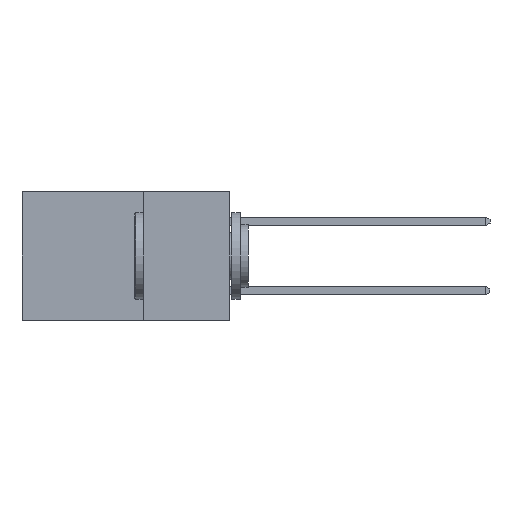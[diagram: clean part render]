
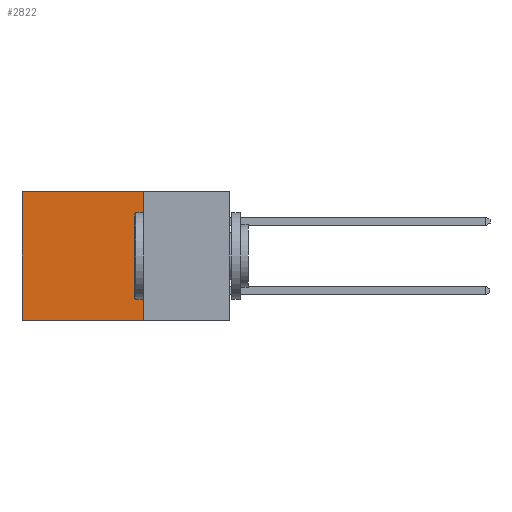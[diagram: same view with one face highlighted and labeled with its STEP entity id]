
A CAD part, left-side view. The second image highlights one B-rep face of the part: STEP entity #2822.
In plain terms, the highlighted planar face has unit normal (-1, 0, 0).
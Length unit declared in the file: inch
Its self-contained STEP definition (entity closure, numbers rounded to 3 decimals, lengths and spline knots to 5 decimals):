
#36 = VERTEX_POINT ( 'NONE', #3144 ) ;
#162 = VECTOR ( 'NONE', #6749, 39.37008 ) ;
#214 = PLANE ( 'NONE',  #12803 ) ;
#252 = VECTOR ( 'NONE', #15217, 39.37008 ) ;
#682 = LINE ( 'NONE', #11421, #252 ) ;
#1106 = DIRECTION ( 'NONE',  ( 0., 1., 0. ) ) ;
#1828 = EDGE_CURVE ( 'NONE', #15604, #36, #682, .T. ) ;
#1905 = ORIENTED_EDGE ( 'NONE', *, *, #1828, .T. ) ;
#1920 = ORIENTED_EDGE ( 'NONE', *, *, #9189, .F. ) ;
#2077 = ORIENTED_EDGE ( 'NONE', *, *, #14014, .F. ) ;
#2168 = ORIENTED_EDGE ( 'NONE', *, *, #11996, .T. ) ;
#2822 = ADVANCED_FACE ( 'NONE', ( #4790 ), #214, .F. ) ;
#3144 = CARTESIAN_POINT ( 'NONE',  ( 0.298, 0.6, -0.37 ) ) ;
#4115 = LINE ( 'NONE', #10727, #162 ) ;
#4790 = FACE_OUTER_BOUND ( 'NONE', #11016, .T. ) ;
#5184 = VECTOR ( 'NONE', #1106, 39.37008 ) ;
#5699 = CARTESIAN_POINT ( 'NONE',  ( 0.298, 0.25, 0. ) ) ;
#6082 = CARTESIAN_POINT ( 'NONE',  ( 0.298, 0.25, 0. ) ) ;
#6140 = LINE ( 'NONE', #6082, #13232 ) ;
#6614 = CARTESIAN_POINT ( 'NONE',  ( 0.298, 0.25, 0. ) ) ;
#6749 = DIRECTION ( 'NONE',  ( 0., 1., 0. ) ) ;
#8694 = LINE ( 'NONE', #11652, #5184 ) ;
#8812 = VERTEX_POINT ( 'NONE', #5699 ) ;
#9189 = EDGE_CURVE ( 'NONE', #11630, #36, #4115, .T. ) ;
#10225 = CARTESIAN_POINT ( 'NONE',  ( 0.298, 0.6, 0. ) ) ;
#10727 = CARTESIAN_POINT ( 'NONE',  ( 0.298, 0.25, -0.37 ) ) ;
#11016 = EDGE_LOOP ( 'NONE', ( #1905, #1920, #2077, #2168 ) ) ;
#11421 = CARTESIAN_POINT ( 'NONE',  ( 0.298, 0.6, 0. ) ) ;
#11630 = VERTEX_POINT ( 'NONE', #14070 ) ;
#11652 = CARTESIAN_POINT ( 'NONE',  ( 0.298, 0.25, 0. ) ) ;
#11996 = EDGE_CURVE ( 'NONE', #8812, #15604, #8694, .T. ) ;
#12803 = AXIS2_PLACEMENT_3D ( 'NONE', #6614, #13931, #13946 ) ;
#13232 = VECTOR ( 'NONE', #14069, 39.37008 ) ;
#13931 = DIRECTION ( 'NONE',  ( 1., 0., 0. ) ) ;
#13946 = DIRECTION ( 'NONE',  ( 0., 0., -1. ) ) ;
#14014 = EDGE_CURVE ( 'NONE', #8812, #11630, #6140, .T. ) ;
#14069 = DIRECTION ( 'NONE',  ( 0., 0., -1. ) ) ;
#14070 = CARTESIAN_POINT ( 'NONE',  ( 0.298, 0.25, -0.37 ) ) ;
#15217 = DIRECTION ( 'NONE',  ( 0., 0., -1. ) ) ;
#15604 = VERTEX_POINT ( 'NONE', #10225 ) ;
